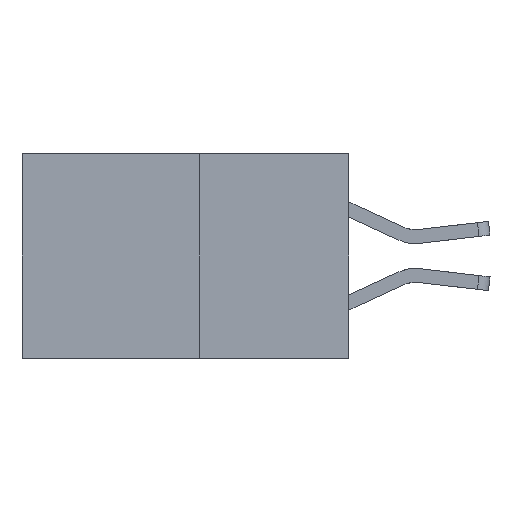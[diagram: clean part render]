
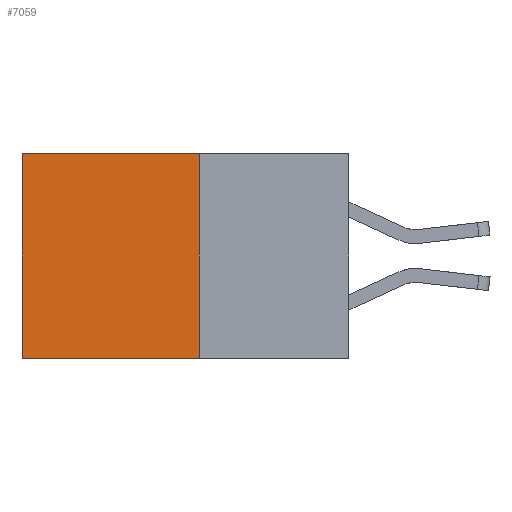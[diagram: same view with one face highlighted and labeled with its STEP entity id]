
A CAD part, left-side view. The second image highlights one B-rep face of the part: STEP entity #7059.
In plain terms, the highlighted planar face has unit normal (-1, 0, 0).
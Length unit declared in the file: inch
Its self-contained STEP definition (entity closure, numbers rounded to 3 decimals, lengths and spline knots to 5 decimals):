
#19 = ORIENTED_EDGE ( 'NONE', *, *, #1825, .T. ) ;
#301 = VECTOR ( 'NONE', #6705, 39.37008 ) ;
#749 = CARTESIAN_POINT ( 'NONE',  ( 0.277, 0.27, 0. ) ) ;
#1227 = VERTEX_POINT ( 'NONE', #9410 ) ;
#1317 = VECTOR ( 'NONE', #6632, 39.37008 ) ;
#1825 = EDGE_CURVE ( 'NONE', #5971, #7214, #3107, .T. ) ;
#2357 = EDGE_CURVE ( 'NONE', #5971, #1227, #10410, .T. ) ;
#2815 = VECTOR ( 'NONE', #6721, 39.37008 ) ;
#3107 = LINE ( 'NONE', #3255, #2815 ) ;
#3255 = CARTESIAN_POINT ( 'NONE',  ( 0.277, 0.27, 0. ) ) ;
#4098 = ORIENTED_EDGE ( 'NONE', *, *, #7497, .T. ) ;
#4124 = LINE ( 'NONE', #7379, #1317 ) ;
#5172 = CARTESIAN_POINT ( 'NONE',  ( 0.277, 0.27, -0.37 ) ) ;
#5421 = CARTESIAN_POINT ( 'NONE',  ( 0.277, 0.59, -0.37 ) ) ;
#5971 = VERTEX_POINT ( 'NONE', #749 ) ;
#6062 = VERTEX_POINT ( 'NONE', #5421 ) ;
#6401 = DIRECTION ( 'NONE',  ( 0., 0., -1. ) ) ;
#6623 = LINE ( 'NONE', #11290, #8875 ) ;
#6632 = DIRECTION ( 'NONE',  ( 0., 1., 0. ) ) ;
#6705 = DIRECTION ( 'NONE',  ( 0., 0., -1. ) ) ;
#6721 = DIRECTION ( 'NONE',  ( 0., 1., 0. ) ) ;
#7059 = ADVANCED_FACE ( 'NONE', ( #8888 ), #8483, .F. ) ;
#7091 = EDGE_CURVE ( 'NONE', #1227, #6062, #4124, .T. ) ;
#7214 = VERTEX_POINT ( 'NONE', #11437 ) ;
#7379 = CARTESIAN_POINT ( 'NONE',  ( 0.277, 0.27, -0.37 ) ) ;
#7401 = AXIS2_PLACEMENT_3D ( 'NONE', #5172, #11970, #6401 ) ;
#7497 = EDGE_CURVE ( 'NONE', #7214, #6062, #6623, .T. ) ;
#7557 = CARTESIAN_POINT ( 'NONE',  ( 0.277, 0.27, -0.37 ) ) ;
#8483 = PLANE ( 'NONE',  #7401 ) ;
#8875 = VECTOR ( 'NONE', #12125, 39.37008 ) ;
#8888 = FACE_OUTER_BOUND ( 'NONE', #12073, .T. ) ;
#9410 = CARTESIAN_POINT ( 'NONE',  ( 0.277, 0.27, -0.37 ) ) ;
#10395 = ORIENTED_EDGE ( 'NONE', *, *, #2357, .F. ) ;
#10410 = LINE ( 'NONE', #7557, #301 ) ;
#11135 = ORIENTED_EDGE ( 'NONE', *, *, #7091, .F. ) ;
#11290 = CARTESIAN_POINT ( 'NONE',  ( 0.277, 0.59, -0.37 ) ) ;
#11437 = CARTESIAN_POINT ( 'NONE',  ( 0.277, 0.59, 0. ) ) ;
#11970 = DIRECTION ( 'NONE',  ( 1., 0., 0. ) ) ;
#12073 = EDGE_LOOP ( 'NONE', ( #4098, #11135, #10395, #19 ) ) ;
#12125 = DIRECTION ( 'NONE',  ( 0., 0., -1. ) ) ;
